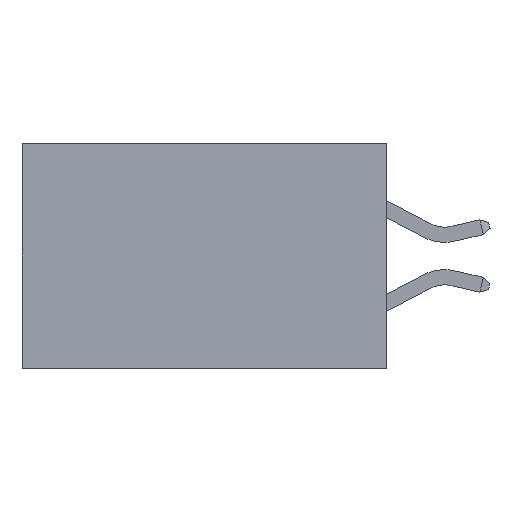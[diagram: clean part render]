
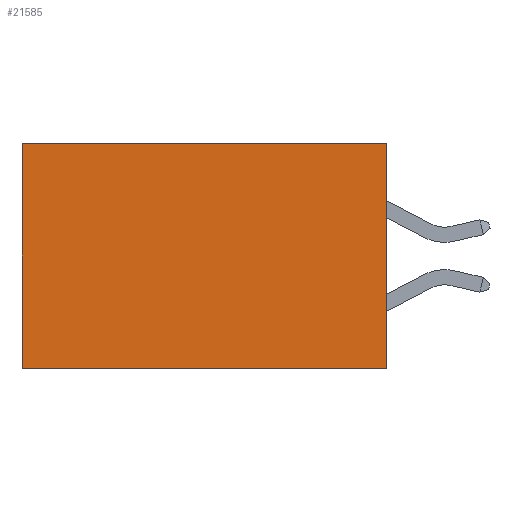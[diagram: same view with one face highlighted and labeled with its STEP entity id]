
A CAD part, left-side view. The second image highlights one B-rep face of the part: STEP entity #21585.
In plain terms, the highlighted planar face has unit normal (-1, 0, 0).
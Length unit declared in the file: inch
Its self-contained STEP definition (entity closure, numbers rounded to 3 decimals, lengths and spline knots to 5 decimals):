
#1081 = DIRECTION ( 'NONE',  ( 1., 0., 0. ) ) ;
#1337 = VECTOR ( 'NONE', #6186, 39.37008 ) ;
#1742 = EDGE_LOOP ( 'NONE', ( #4028, #9872, #3933, #15212 ) ) ;
#2309 = DIRECTION ( 'NONE',  ( 0., 0., -1. ) ) ;
#2628 = CARTESIAN_POINT ( 'NONE',  ( 0.298, 0., -0.37 ) ) ;
#2662 = CARTESIAN_POINT ( 'NONE',  ( 0.298, 0.6, 0. ) ) ;
#2687 = LINE ( 'NONE', #7941, #16624 ) ;
#2743 = LINE ( 'NONE', #2628, #18817 ) ;
#3933 = ORIENTED_EDGE ( 'NONE', *, *, #6883, .F. ) ;
#4028 = ORIENTED_EDGE ( 'NONE', *, *, #22260, .T. ) ;
#4551 = DIRECTION ( 'NONE',  ( 0., 1., 0. ) ) ;
#4813 = FACE_OUTER_BOUND ( 'NONE', #1742, .T. ) ;
#6186 = DIRECTION ( 'NONE',  ( 0., 0., -1. ) ) ;
#6377 = LINE ( 'NONE', #16383, #1337 ) ;
#6883 = EDGE_CURVE ( 'NONE', #21162, #20553, #6377, .T. ) ;
#7941 = CARTESIAN_POINT ( 'NONE',  ( 0.298, 0.6, 0. ) ) ;
#9872 = ORIENTED_EDGE ( 'NONE', *, *, #18859, .F. ) ;
#10684 = AXIS2_PLACEMENT_3D ( 'NONE', #12173, #1081, #13969 ) ;
#11217 = CARTESIAN_POINT ( 'NONE',  ( 0.298, 0., -0.37 ) ) ;
#11800 = VERTEX_POINT ( 'NONE', #2662 ) ;
#12096 = DIRECTION ( 'NONE',  ( 0., 1., 0. ) ) ;
#12173 = CARTESIAN_POINT ( 'NONE',  ( 0.298, 0., 0. ) ) ;
#12823 = CARTESIAN_POINT ( 'NONE',  ( 0.298, 0., 0. ) ) ;
#12851 = LINE ( 'NONE', #22677, #22785 ) ;
#13969 = DIRECTION ( 'NONE',  ( 0., 0., -1. ) ) ;
#14227 = CARTESIAN_POINT ( 'NONE',  ( 0.298, 0.6, -0.37 ) ) ;
#15212 = ORIENTED_EDGE ( 'NONE', *, *, #19631, .T. ) ;
#16383 = CARTESIAN_POINT ( 'NONE',  ( 0.298, 0., 0. ) ) ;
#16624 = VECTOR ( 'NONE', #2309, 39.37008 ) ;
#18817 = VECTOR ( 'NONE', #4551, 39.37008 ) ;
#18859 = EDGE_CURVE ( 'NONE', #20553, #21035, #2743, .T. ) ;
#19631 = EDGE_CURVE ( 'NONE', #21162, #11800, #12851, .T. ) ;
#20553 = VERTEX_POINT ( 'NONE', #11217 ) ;
#21003 = PLANE ( 'NONE',  #10684 ) ;
#21035 = VERTEX_POINT ( 'NONE', #14227 ) ;
#21162 = VERTEX_POINT ( 'NONE', #12823 ) ;
#21585 = ADVANCED_FACE ( 'NONE', ( #4813 ), #21003, .F. ) ;
#22260 = EDGE_CURVE ( 'NONE', #11800, #21035, #2687, .T. ) ;
#22677 = CARTESIAN_POINT ( 'NONE',  ( 0.298, 0., 0. ) ) ;
#22785 = VECTOR ( 'NONE', #12096, 39.37008 ) ;
